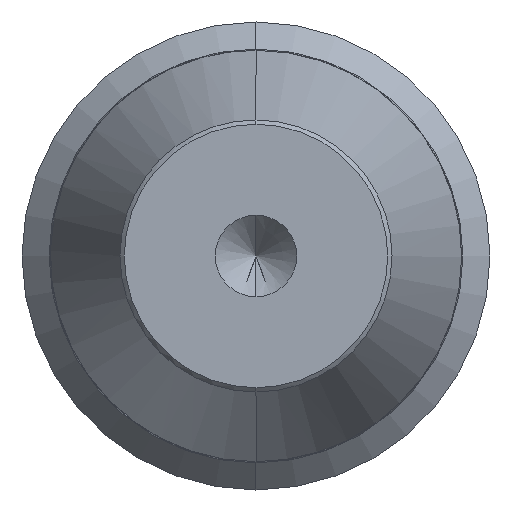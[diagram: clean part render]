
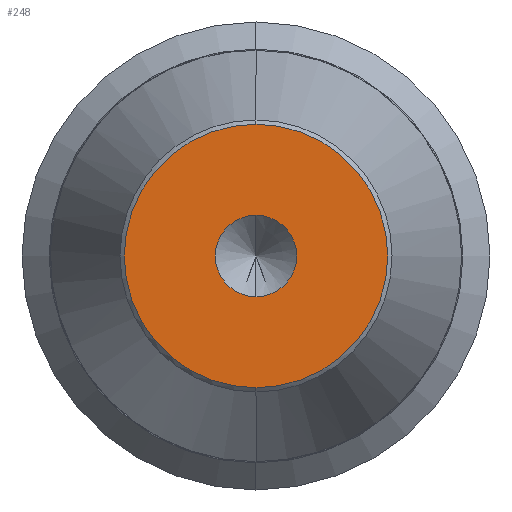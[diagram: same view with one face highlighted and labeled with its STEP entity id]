
A CAD part, left-side view. The second image highlights one B-rep face of the part: STEP entity #248.
In plain terms, the highlighted planar face has unit normal (-1, 0, 0).
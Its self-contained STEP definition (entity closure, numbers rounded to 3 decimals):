
#26 = ORIENTED_EDGE ( 'NONE', *, *, #325, .F. ) ;
#33 = DIRECTION ( 'NONE',  ( 0., 0., -1. ) ) ;
#44 = CARTESIAN_POINT ( 'NONE',  ( -114.21, 46.514, -0.65 ) ) ;
#77 = DIRECTION ( 'NONE',  ( 1., 0., 0. ) ) ;
#134 = AXIS2_PLACEMENT_3D ( 'NONE', #523, #214, #447 ) ;
#156 = DIRECTION ( 'NONE',  ( 0., 0., -1. ) ) ;
#188 = EDGE_LOOP ( 'NONE', ( #26, #347 ) ) ;
#214 = DIRECTION ( 'NONE',  ( -1., 0., 0. ) ) ;
#245 = PLANE ( 'NONE',  #639 ) ;
#248 = ADVANCED_FACE ( 'NONE', ( #1042, #472 ), #245, .F. ) ;
#270 = DIRECTION ( 'NONE',  ( 1., 0., 0. ) ) ;
#325 = EDGE_CURVE ( 'NONE', #958, #884, #659, .T. ) ;
#343 = EDGE_CURVE ( 'NONE', #441, #382, #926, .T. ) ;
#347 = ORIENTED_EDGE ( 'NONE', *, *, #873, .F. ) ;
#352 = CIRCLE ( 'NONE', #506, 5.35 ) ;
#363 = CARTESIAN_POINT ( 'NONE',  ( -114.21, 46.514, 1. ) ) ;
#382 = VERTEX_POINT ( 'NONE', #973 ) ;
#409 = CARTESIAN_POINT ( 'NONE',  ( -114.21, 46.514, 1. ) ) ;
#429 = DIRECTION ( 'NONE',  ( 1., 0., 0. ) ) ;
#441 = VERTEX_POINT ( 'NONE', #44 ) ;
#447 = DIRECTION ( 'NONE',  ( 0., 0., 1. ) ) ;
#472 = FACE_OUTER_BOUND ( 'NONE', #188, .T. ) ;
#506 = AXIS2_PLACEMENT_3D ( 'NONE', #363, #429, #33 ) ;
#510 = CARTESIAN_POINT ( 'NONE',  ( -114.21, 46.514, 1. ) ) ;
#523 = CARTESIAN_POINT ( 'NONE',  ( -114.21, 46.514, 1. ) ) ;
#536 = ORIENTED_EDGE ( 'NONE', *, *, #343, .F. ) ;
#571 = CIRCLE ( 'NONE', #134, 1.65 ) ;
#576 = DIRECTION ( 'NONE',  ( -1., 0., 0. ) ) ;
#582 = DIRECTION ( 'NONE',  ( 0., 0., -1. ) ) ;
#586 = AXIS2_PLACEMENT_3D ( 'NONE', #510, #576, #983 ) ;
#639 = AXIS2_PLACEMENT_3D ( 'NONE', #723, #77, #156 ) ;
#659 = CIRCLE ( 'NONE', #1005, 5.35 ) ;
#689 = EDGE_LOOP ( 'NONE', ( #756, #536 ) ) ;
#723 = CARTESIAN_POINT ( 'NONE',  ( -114.21, 46.514, 9.35 ) ) ;
#756 = ORIENTED_EDGE ( 'NONE', *, *, #766, .F. ) ;
#766 = EDGE_CURVE ( 'NONE', #382, #441, #571, .T. ) ;
#798 = CARTESIAN_POINT ( 'NONE',  ( -114.21, 46.514, -4.35 ) ) ;
#873 = EDGE_CURVE ( 'NONE', #884, #958, #352, .T. ) ;
#884 = VERTEX_POINT ( 'NONE', #917 ) ;
#917 = CARTESIAN_POINT ( 'NONE',  ( -114.21, 46.514, 6.35 ) ) ;
#926 = CIRCLE ( 'NONE', #586, 1.65 ) ;
#958 = VERTEX_POINT ( 'NONE', #798 ) ;
#973 = CARTESIAN_POINT ( 'NONE',  ( -114.21, 46.514, 2.65 ) ) ;
#983 = DIRECTION ( 'NONE',  ( 0., 0., 1. ) ) ;
#1005 = AXIS2_PLACEMENT_3D ( 'NONE', #409, #270, #582 ) ;
#1042 = FACE_BOUND ( 'NONE', #689, .T. ) ;
